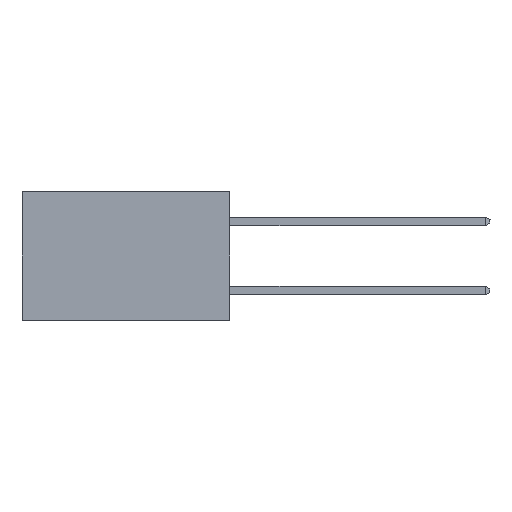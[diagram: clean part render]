
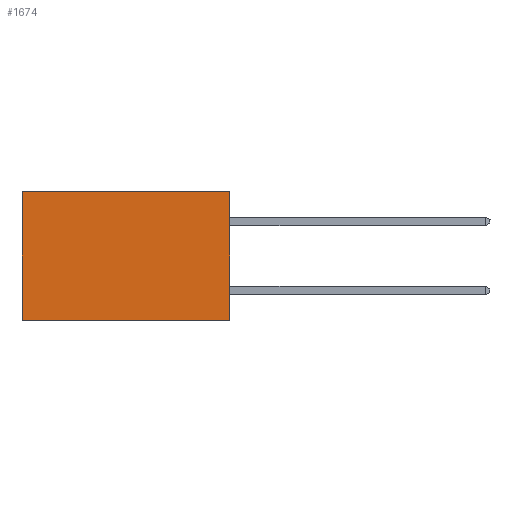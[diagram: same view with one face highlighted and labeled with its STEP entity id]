
A CAD part, left-side view. The second image highlights one B-rep face of the part: STEP entity #1674.
In plain terms, the highlighted planar face has unit normal (-1, 0, 0).
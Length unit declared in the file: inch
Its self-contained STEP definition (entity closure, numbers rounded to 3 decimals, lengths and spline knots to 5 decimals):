
#46 = EDGE_CURVE ( 'NONE', #2025, #5964, #7088, .T. ) ;
#490 = CARTESIAN_POINT ( 'NONE',  ( 0.298, 0.6, 0. ) ) ;
#671 = CARTESIAN_POINT ( 'NONE',  ( 0.298, 0., 0. ) ) ;
#865 = CARTESIAN_POINT ( 'NONE',  ( 0.298, 0., 0. ) ) ;
#1091 = VECTOR ( 'NONE', #5545, 39.37008 ) ;
#1144 = DIRECTION ( 'NONE',  ( 0., 0., -1. ) ) ;
#1325 = AXIS2_PLACEMENT_3D ( 'NONE', #2399, #7292, #1144 ) ;
#1413 = VERTEX_POINT ( 'NONE', #865 ) ;
#1487 = EDGE_LOOP ( 'NONE', ( #4370, #8858, #1499, #1824 ) ) ;
#1499 = ORIENTED_EDGE ( 'NONE', *, *, #3263, .F. ) ;
#1532 = CARTESIAN_POINT ( 'NONE',  ( 0.298, 0.6, 0. ) ) ;
#1674 = ADVANCED_FACE ( 'NONE', ( #2836 ), #6650, .F. ) ;
#1776 = CARTESIAN_POINT ( 'NONE',  ( 0.298, 0., -0.37 ) ) ;
#1824 = ORIENTED_EDGE ( 'NONE', *, *, #1945, .T. ) ;
#1945 = EDGE_CURVE ( 'NONE', #1413, #2025, #6165, .T. ) ;
#2025 = VERTEX_POINT ( 'NONE', #1532 ) ;
#2230 = DIRECTION ( 'NONE',  ( 0., 0., -1. ) ) ;
#2399 = CARTESIAN_POINT ( 'NONE',  ( 0.298, 0., 0. ) ) ;
#2503 = DIRECTION ( 'NONE',  ( 0., 0., -1. ) ) ;
#2521 = EDGE_CURVE ( 'NONE', #7085, #5964, #3655, .T. ) ;
#2836 = FACE_OUTER_BOUND ( 'NONE', #1487, .T. ) ;
#2966 = VECTOR ( 'NONE', #2230, 39.37008 ) ;
#3248 = CARTESIAN_POINT ( 'NONE',  ( 0.298, 0., 0. ) ) ;
#3263 = EDGE_CURVE ( 'NONE', #1413, #7085, #7831, .T. ) ;
#3655 = LINE ( 'NONE', #6990, #1091 ) ;
#3959 = VECTOR ( 'NONE', #2503, 39.37008 ) ;
#4370 = ORIENTED_EDGE ( 'NONE', *, *, #46, .T. ) ;
#4994 = CARTESIAN_POINT ( 'NONE',  ( 0.298, 0.6, -0.37 ) ) ;
#5545 = DIRECTION ( 'NONE',  ( 0., 1., 0. ) ) ;
#5964 = VERTEX_POINT ( 'NONE', #4994 ) ;
#6165 = LINE ( 'NONE', #671, #8083 ) ;
#6650 = PLANE ( 'NONE',  #1325 ) ;
#6990 = CARTESIAN_POINT ( 'NONE',  ( 0.298, 0., -0.37 ) ) ;
#7085 = VERTEX_POINT ( 'NONE', #1776 ) ;
#7088 = LINE ( 'NONE', #490, #2966 ) ;
#7292 = DIRECTION ( 'NONE',  ( 1., 0., 0. ) ) ;
#7831 = LINE ( 'NONE', #3248, #3959 ) ;
#8083 = VECTOR ( 'NONE', #8282, 39.37008 ) ;
#8282 = DIRECTION ( 'NONE',  ( 0., 1., 0. ) ) ;
#8858 = ORIENTED_EDGE ( 'NONE', *, *, #2521, .F. ) ;
